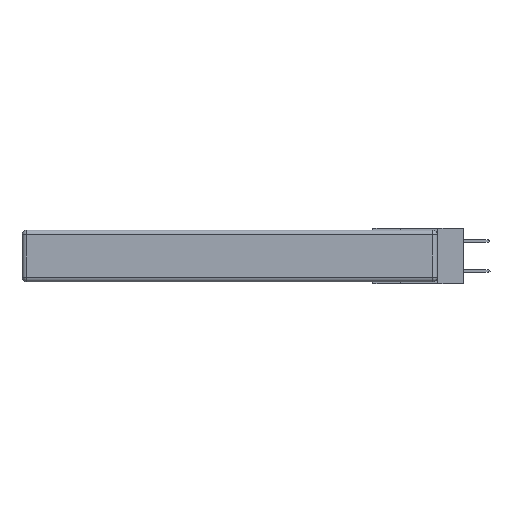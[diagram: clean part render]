
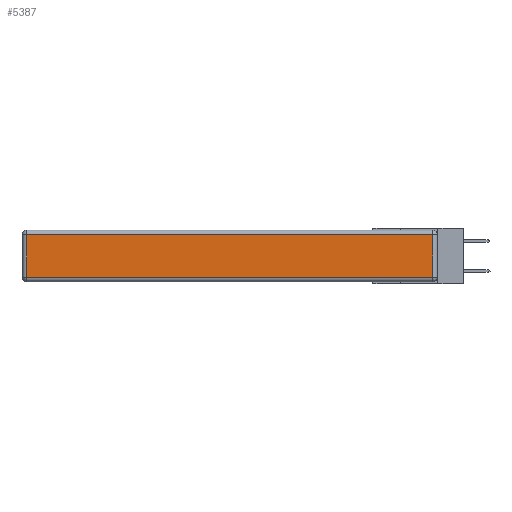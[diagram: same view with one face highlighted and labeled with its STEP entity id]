
A CAD part, left-side view. The second image highlights one B-rep face of the part: STEP entity #5387.
In plain terms, the highlighted planar face has unit normal (-1, 0, 0).
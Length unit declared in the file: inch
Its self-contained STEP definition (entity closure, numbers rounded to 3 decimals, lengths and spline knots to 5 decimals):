
#5 = CARTESIAN_POINT ( 'NONE',  ( 0., 0.03, -0.313 ) ) ;
#780 = VECTOR ( 'NONE', #9576, 39.37008 ) ;
#1166 = CARTESIAN_POINT ( 'NONE',  ( 0., 0., -0.313 ) ) ;
#1267 = LINE ( 'NONE', #8274, #1755 ) ;
#1288 = ORIENTED_EDGE ( 'NONE', *, *, #10125, .T. ) ;
#1713 = VERTEX_POINT ( 'NONE', #13383 ) ;
#1755 = VECTOR ( 'NONE', #3048, 39.37008 ) ;
#2198 = EDGE_CURVE ( 'NONE', #11829, #6719, #1267, .T. ) ;
#2275 = EDGE_CURVE ( 'NONE', #6719, #5950, #8482, .T. ) ;
#2511 = DIRECTION ( 'NONE',  ( 0., 1., 0. ) ) ;
#2591 = CARTESIAN_POINT ( 'NONE',  ( 0., 0., -0.343 ) ) ;
#2606 = EDGE_CURVE ( 'NONE', #1713, #11829, #5884, .T. ) ;
#3048 = DIRECTION ( 'NONE',  ( 0., 0., -1. ) ) ;
#4136 = EDGE_LOOP ( 'NONE', ( #13474, #1288, #5696, #6097 ) ) ;
#5387 = ADVANCED_FACE ( 'NONE', ( #12025 ), #11650, .T. ) ;
#5546 = CARTESIAN_POINT ( 'NONE',  ( 0., 0.03, -0.343 ) ) ;
#5696 = ORIENTED_EDGE ( 'NONE', *, *, #2606, .T. ) ;
#5798 = LINE ( 'NONE', #5546, #11050 ) ;
#5884 = LINE ( 'NONE', #12890, #7983 ) ;
#5950 = VERTEX_POINT ( 'NONE', #5 ) ;
#6097 = ORIENTED_EDGE ( 'NONE', *, *, #2198, .T. ) ;
#6532 = DIRECTION ( 'NONE',  ( 0., 0., 1. ) ) ;
#6719 = VERTEX_POINT ( 'NONE', #7038 ) ;
#6723 = DIRECTION ( 'NONE',  ( -1., 0., 0. ) ) ;
#7038 = CARTESIAN_POINT ( 'NONE',  ( 0., 2.72, -0.313 ) ) ;
#7983 = VECTOR ( 'NONE', #2511, 39.37008 ) ;
#8056 = CARTESIAN_POINT ( 'NONE',  ( 0., 2.72, -0.03 ) ) ;
#8274 = CARTESIAN_POINT ( 'NONE',  ( 0., 2.72, -0.343 ) ) ;
#8482 = LINE ( 'NONE', #1166, #780 ) ;
#9576 = DIRECTION ( 'NONE',  ( 0., -1., 0. ) ) ;
#10125 = EDGE_CURVE ( 'NONE', #5950, #1713, #5798, .T. ) ;
#10958 = AXIS2_PLACEMENT_3D ( 'NONE', #2591, #6723, #13196 ) ;
#11050 = VECTOR ( 'NONE', #6532, 39.37008 ) ;
#11650 = PLANE ( 'NONE',  #10958 ) ;
#11829 = VERTEX_POINT ( 'NONE', #8056 ) ;
#12025 = FACE_OUTER_BOUND ( 'NONE', #4136, .T. ) ;
#12890 = CARTESIAN_POINT ( 'NONE',  ( 0., 2.75, -0.03 ) ) ;
#13196 = DIRECTION ( 'NONE',  ( 0., 0., 1. ) ) ;
#13383 = CARTESIAN_POINT ( 'NONE',  ( 0., 0.03, -0.03 ) ) ;
#13474 = ORIENTED_EDGE ( 'NONE', *, *, #2275, .T. ) ;
